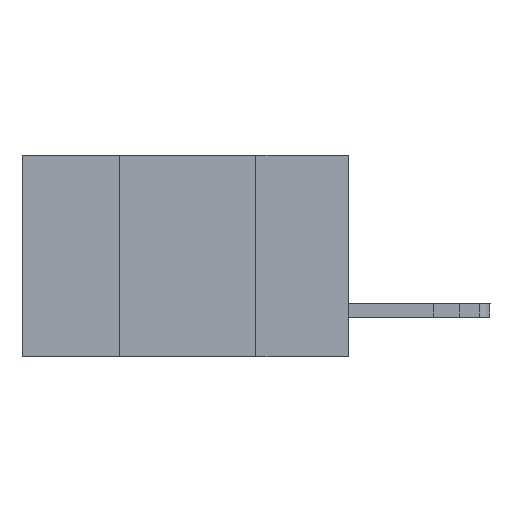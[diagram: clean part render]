
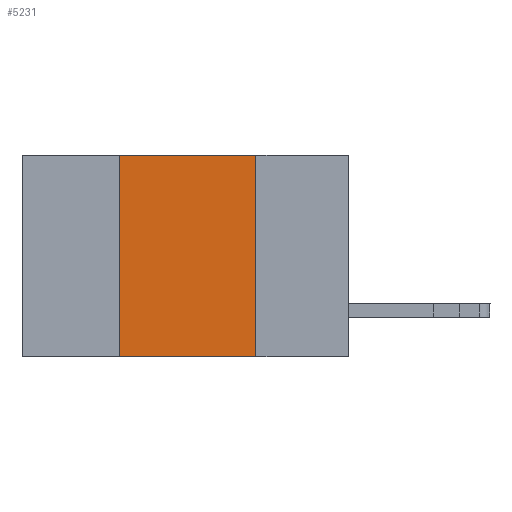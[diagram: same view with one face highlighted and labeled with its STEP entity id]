
A CAD part, left-side view. The second image highlights one B-rep face of the part: STEP entity #5231.
In plain terms, the highlighted planar face has unit normal (-1, 0, 0).
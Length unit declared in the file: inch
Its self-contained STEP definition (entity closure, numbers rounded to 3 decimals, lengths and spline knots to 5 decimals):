
#31 = DIRECTION ( 'NONE',  ( 0., 0., 1. ) ) ;
#167 = LINE ( 'NONE', #12475, #6209 ) ;
#203 = CARTESIAN_POINT ( 'NONE',  ( 0., 0.42, -0.37 ) ) ;
#230 = ORIENTED_EDGE ( 'NONE', *, *, #10368, .F. ) ;
#944 = EDGE_LOOP ( 'NONE', ( #2887, #230, #1884, #8853 ) ) ;
#1653 = PLANE ( 'NONE',  #13174 ) ;
#1884 = ORIENTED_EDGE ( 'NONE', *, *, #8802, .F. ) ;
#2441 = CARTESIAN_POINT ( 'NONE',  ( 0., 0.6, -0.37 ) ) ;
#2843 = EDGE_CURVE ( 'NONE', #5966, #5972, #8189, .T. ) ;
#2887 = ORIENTED_EDGE ( 'NONE', *, *, #2843, .F. ) ;
#3228 = LINE ( 'NONE', #2441, #12323 ) ;
#3772 = CARTESIAN_POINT ( 'NONE',  ( 0., 0.17, 0. ) ) ;
#3905 = VERTEX_POINT ( 'NONE', #203 ) ;
#4316 = CARTESIAN_POINT ( 'NONE',  ( 0., 0.42, 0. ) ) ;
#4913 = CARTESIAN_POINT ( 'NONE',  ( 0., 0.17, 0. ) ) ;
#5231 = ADVANCED_FACE ( 'NONE', ( #10361 ), #1653, .F. ) ;
#5966 = VERTEX_POINT ( 'NONE', #3772 ) ;
#5972 = VERTEX_POINT ( 'NONE', #10875 ) ;
#6209 = VECTOR ( 'NONE', #10398, 39.37008 ) ;
#6253 = VECTOR ( 'NONE', #31, 39.37008 ) ;
#6825 = DIRECTION ( 'NONE',  ( 0., 0., -1. ) ) ;
#6909 = CARTESIAN_POINT ( 'NONE',  ( 0., 0.6, 0. ) ) ;
#8189 = LINE ( 'NONE', #4913, #13259 ) ;
#8802 = EDGE_CURVE ( 'NONE', #3905, #12385, #11271, .T. ) ;
#8853 = ORIENTED_EDGE ( 'NONE', *, *, #12529, .T. ) ;
#10361 = FACE_OUTER_BOUND ( 'NONE', #944, .T. ) ;
#10368 = EDGE_CURVE ( 'NONE', #12385, #5966, #167, .T. ) ;
#10398 = DIRECTION ( 'NONE',  ( 0., -1., 0. ) ) ;
#10812 = DIRECTION ( 'NONE',  ( 0., -1., 0. ) ) ;
#10875 = CARTESIAN_POINT ( 'NONE',  ( 0., 0.17, -0.37 ) ) ;
#11114 = DIRECTION ( 'NONE',  ( 1., 0., 0. ) ) ;
#11271 = LINE ( 'NONE', #13375, #6253 ) ;
#12066 = DIRECTION ( 'NONE',  ( 0., 0., -1. ) ) ;
#12323 = VECTOR ( 'NONE', #10812, 39.37008 ) ;
#12385 = VERTEX_POINT ( 'NONE', #4316 ) ;
#12475 = CARTESIAN_POINT ( 'NONE',  ( 0., 0.6, 0. ) ) ;
#12529 = EDGE_CURVE ( 'NONE', #3905, #5972, #3228, .T. ) ;
#13174 = AXIS2_PLACEMENT_3D ( 'NONE', #6909, #11114, #6825 ) ;
#13259 = VECTOR ( 'NONE', #12066, 39.37008 ) ;
#13375 = CARTESIAN_POINT ( 'NONE',  ( 0., 0.42, 0. ) ) ;
